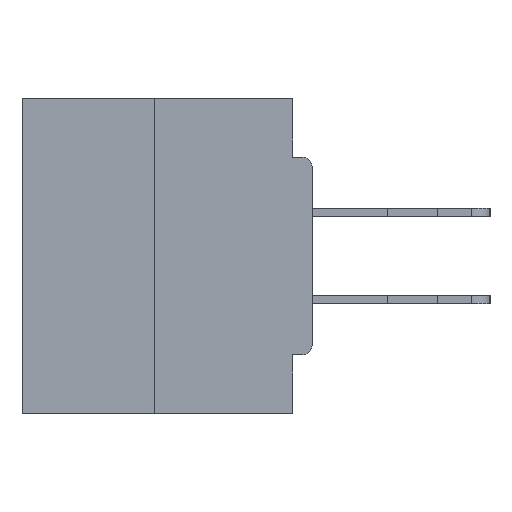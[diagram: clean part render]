
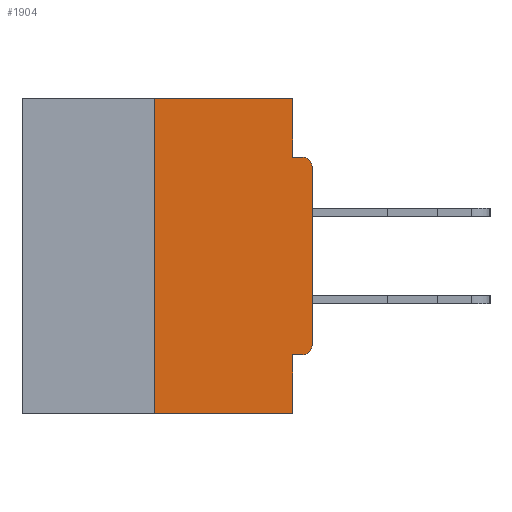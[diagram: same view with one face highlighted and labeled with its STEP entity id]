
A CAD part, left-side view. The second image highlights one B-rep face of the part: STEP entity #1904.
In plain terms, the highlighted planar face has unit normal (-1, 0, 0).
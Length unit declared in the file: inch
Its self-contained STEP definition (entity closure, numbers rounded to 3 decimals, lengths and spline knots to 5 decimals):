
#74 = VECTOR ( 'NONE', #18704, 39.37008 ) ;
#276 = LINE ( 'NONE', #25319, #27682 ) ;
#345 = EDGE_CURVE ( 'NONE', #24942, #26765, #276, .T. ) ;
#569 = DIRECTION ( 'NONE',  ( 0., 0., -1. ) ) ;
#1634 = EDGE_LOOP ( 'NONE', ( #15955, #24776, #9263, #8293, #2030, #21764, #7105, #31456, #28863, #27032 ) ) ;
#1641 = DIRECTION ( 'NONE',  ( -1., 0., 0. ) ) ;
#1904 = ADVANCED_FACE ( 'NONE', ( #31763 ), #26869, .F. ) ;
#2030 = ORIENTED_EDGE ( 'NONE', *, *, #27941, .F. ) ;
#2289 = CARTESIAN_POINT ( 'NONE',  ( 0., 0.25, -0.5 ) ) ;
#2512 = CARTESIAN_POINT ( 'NONE',  ( 0., 0., -0.3915 ) ) ;
#3093 = VECTOR ( 'NONE', #28970, 39.37008 ) ;
#3356 = CARTESIAN_POINT ( 'NONE',  ( 0., 0.46, 0. ) ) ;
#3663 = VERTEX_POINT ( 'NONE', #4790 ) ;
#4225 = VERTEX_POINT ( 'NONE', #2512 ) ;
#4790 = CARTESIAN_POINT ( 'NONE',  ( 0., 0., -0.1085 ) ) ;
#5992 = VECTOR ( 'NONE', #11463, 39.37008 ) ;
#6094 = CARTESIAN_POINT ( 'NONE',  ( 0., 0.015, -0.3915 ) ) ;
#6111 = CARTESIAN_POINT ( 'NONE',  ( 0., 0.25, 0. ) ) ;
#6358 = VECTOR ( 'NONE', #33410, 39.37008 ) ;
#6386 = LINE ( 'NONE', #13212, #74 ) ;
#6655 = CARTESIAN_POINT ( 'NONE',  ( 0., 0.031, -0.4065 ) ) ;
#7105 = ORIENTED_EDGE ( 'NONE', *, *, #33654, .T. ) ;
#8293 = ORIENTED_EDGE ( 'NONE', *, *, #345, .F. ) ;
#8464 = LINE ( 'NONE', #22659, #21989 ) ;
#8552 = DIRECTION ( 'NONE',  ( -1., 0., 0. ) ) ;
#9263 = ORIENTED_EDGE ( 'NONE', *, *, #32339, .T. ) ;
#9475 = DIRECTION ( 'NONE',  ( 0., 0., -1. ) ) ;
#9731 = CARTESIAN_POINT ( 'NONE',  ( 0., 0.25, 0. ) ) ;
#9865 = CARTESIAN_POINT ( 'NONE',  ( 0., 0.015, -0.1085 ) ) ;
#10654 = CARTESIAN_POINT ( 'NONE',  ( 0., 0.031, -0.5 ) ) ;
#11436 = CIRCLE ( 'NONE', #28475, 0.015 ) ;
#11463 = DIRECTION ( 'NONE',  ( 0., -1., 0. ) ) ;
#12848 = CARTESIAN_POINT ( 'NONE',  ( 0., 0.46, -0.5 ) ) ;
#13212 = CARTESIAN_POINT ( 'NONE',  ( 0., 0., -0.0935 ) ) ;
#13966 = LINE ( 'NONE', #3356, #5992 ) ;
#14524 = EDGE_CURVE ( 'NONE', #21929, #17546, #13966, .T. ) ;
#15197 = LINE ( 'NONE', #26909, #21521 ) ;
#15455 = CARTESIAN_POINT ( 'NONE',  ( 0., 0.031, 0. ) ) ;
#15955 = ORIENTED_EDGE ( 'NONE', *, *, #14524, .F. ) ;
#16143 = LINE ( 'NONE', #12848, #3093 ) ;
#16391 = DIRECTION ( 'NONE',  ( 0., 1., 0. ) ) ;
#16671 = CARTESIAN_POINT ( 'NONE',  ( 0., 0.031, 0. ) ) ;
#17180 = CARTESIAN_POINT ( 'NONE',  ( 0., 0.015, -0.4065 ) ) ;
#17283 = EDGE_CURVE ( 'NONE', #3663, #29900, #11436, .T. ) ;
#17546 = VERTEX_POINT ( 'NONE', #15455 ) ;
#17665 = DIRECTION ( 'NONE',  ( 0., 0., 1. ) ) ;
#17798 = EDGE_CURVE ( 'NONE', #30675, #29900, #6386, .T. ) ;
#18704 = DIRECTION ( 'NONE',  ( 0., -1., 0. ) ) ;
#19542 = DIRECTION ( 'NONE',  ( 0., 0., -1. ) ) ;
#20644 = CARTESIAN_POINT ( 'NONE',  ( 0., 0.031, -0.0935 ) ) ;
#21521 = VECTOR ( 'NONE', #16391, 39.37008 ) ;
#21764 = ORIENTED_EDGE ( 'NONE', *, *, #28824, .T. ) ;
#21929 = VERTEX_POINT ( 'NONE', #9731 ) ;
#21989 = VECTOR ( 'NONE', #17665, 39.37008 ) ;
#22380 = CARTESIAN_POINT ( 'NONE',  ( 0., 0.015, -0.0935 ) ) ;
#22659 = CARTESIAN_POINT ( 'NONE',  ( 0., 0., 0. ) ) ;
#22756 = CIRCLE ( 'NONE', #25084, 0.015 ) ;
#23452 = DIRECTION ( 'NONE',  ( 0., 0., -1. ) ) ;
#23687 = LINE ( 'NONE', #6111, #6358 ) ;
#23805 = DIRECTION ( 'NONE',  ( 0., 0., -1. ) ) ;
#24252 = CARTESIAN_POINT ( 'NONE',  ( 0., 0.46, 0. ) ) ;
#24358 = VERTEX_POINT ( 'NONE', #17180 ) ;
#24776 = ORIENTED_EDGE ( 'NONE', *, *, #33565, .F. ) ;
#24942 = VERTEX_POINT ( 'NONE', #6655 ) ;
#25084 = AXIS2_PLACEMENT_3D ( 'NONE', #6094, #8552, #19542 ) ;
#25319 = CARTESIAN_POINT ( 'NONE',  ( 0., 0.031, -0.5 ) ) ;
#26008 = VECTOR ( 'NONE', #569, 39.37008 ) ;
#26765 = VERTEX_POINT ( 'NONE', #10654 ) ;
#26869 = PLANE ( 'NONE',  #27093 ) ;
#26909 = CARTESIAN_POINT ( 'NONE',  ( 0., 0., -0.4065 ) ) ;
#27032 = ORIENTED_EDGE ( 'NONE', *, *, #34602, .F. ) ;
#27093 = AXIS2_PLACEMENT_3D ( 'NONE', #24252, #34567, #23805 ) ;
#27682 = VECTOR ( 'NONE', #9475, 39.37008 ) ;
#27941 = EDGE_CURVE ( 'NONE', #24358, #24942, #15197, .T. ) ;
#28475 = AXIS2_PLACEMENT_3D ( 'NONE', #9865, #1641, #23452 ) ;
#28824 = EDGE_CURVE ( 'NONE', #24358, #4225, #22756, .T. ) ;
#28863 = ORIENTED_EDGE ( 'NONE', *, *, #17798, .F. ) ;
#28970 = DIRECTION ( 'NONE',  ( 0., -1., 0. ) ) ;
#29514 = VERTEX_POINT ( 'NONE', #2289 ) ;
#29778 = LINE ( 'NONE', #16671, #26008 ) ;
#29900 = VERTEX_POINT ( 'NONE', #22380 ) ;
#30675 = VERTEX_POINT ( 'NONE', #20644 ) ;
#31456 = ORIENTED_EDGE ( 'NONE', *, *, #17283, .T. ) ;
#31763 = FACE_OUTER_BOUND ( 'NONE', #1634, .T. ) ;
#32339 = EDGE_CURVE ( 'NONE', #29514, #26765, #16143, .T. ) ;
#33410 = DIRECTION ( 'NONE',  ( 0., 0., 1. ) ) ;
#33565 = EDGE_CURVE ( 'NONE', #29514, #21929, #23687, .T. ) ;
#33654 = EDGE_CURVE ( 'NONE', #4225, #3663, #8464, .T. ) ;
#34567 = DIRECTION ( 'NONE',  ( 1., 0., 0. ) ) ;
#34602 = EDGE_CURVE ( 'NONE', #17546, #30675, #29778, .T. ) ;
